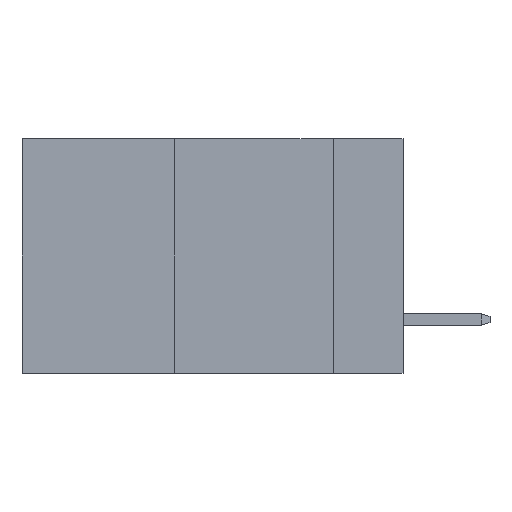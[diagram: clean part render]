
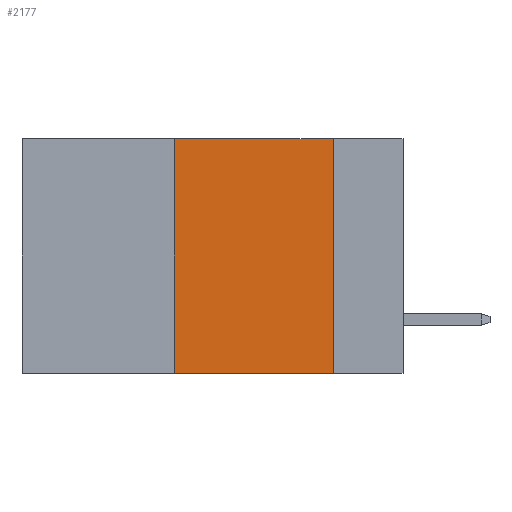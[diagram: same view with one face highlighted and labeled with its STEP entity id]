
A CAD part, left-side view. The second image highlights one B-rep face of the part: STEP entity #2177.
In plain terms, the highlighted planar face has unit normal (-1, 0, 0).
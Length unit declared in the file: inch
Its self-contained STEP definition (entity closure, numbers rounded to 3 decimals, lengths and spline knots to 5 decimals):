
#65 = ORIENTED_EDGE ( 'NONE', *, *, #12275, .F. ) ;
#201 = EDGE_CURVE ( 'NONE', #8243, #3145, #10581, .T. ) ;
#1287 = CARTESIAN_POINT ( 'NONE',  ( 0., 0.36, -0.37 ) ) ;
#1814 = PLANE ( 'NONE',  #11756 ) ;
#1875 = ORIENTED_EDGE ( 'NONE', *, *, #201, .F. ) ;
#1886 = ORIENTED_EDGE ( 'NONE', *, *, #10326, .F. ) ;
#2177 = ADVANCED_FACE ( 'NONE', ( #11460 ), #1814, .F. ) ;
#2230 = EDGE_CURVE ( 'NONE', #8243, #5946, #9363, .T. ) ;
#2442 = CARTESIAN_POINT ( 'NONE',  ( 0., 0.11, 0. ) ) ;
#2740 = VECTOR ( 'NONE', #7527, 39.37008 ) ;
#2976 = CARTESIAN_POINT ( 'NONE',  ( 0., 0.11, 0. ) ) ;
#3145 = VERTEX_POINT ( 'NONE', #3459 ) ;
#3459 = CARTESIAN_POINT ( 'NONE',  ( 0., 0.36, 0. ) ) ;
#4004 = CARTESIAN_POINT ( 'NONE',  ( 0., 0.6, -0.37 ) ) ;
#4870 = ORIENTED_EDGE ( 'NONE', *, *, #2230, .T. ) ;
#4958 = CARTESIAN_POINT ( 'NONE',  ( 0., 0.36, 0. ) ) ;
#5744 = EDGE_LOOP ( 'NONE', ( #65, #1886, #1875, #4870 ) ) ;
#5946 = VERTEX_POINT ( 'NONE', #12658 ) ;
#6119 = CARTESIAN_POINT ( 'NONE',  ( 0., 0.6, 0. ) ) ;
#7527 = DIRECTION ( 'NONE',  ( 0., -1., 0. ) ) ;
#8136 = DIRECTION ( 'NONE',  ( 0., 0., -1. ) ) ;
#8166 = VECTOR ( 'NONE', #8306, 39.37008 ) ;
#8243 = VERTEX_POINT ( 'NONE', #1287 ) ;
#8306 = DIRECTION ( 'NONE',  ( 0., -1., 0. ) ) ;
#8490 = DIRECTION ( 'NONE',  ( 0., 0., 1. ) ) ;
#9363 = LINE ( 'NONE', #4004, #8166 ) ;
#9578 = CARTESIAN_POINT ( 'NONE',  ( 0., 0.6, 0. ) ) ;
#9684 = VECTOR ( 'NONE', #8490, 39.37008 ) ;
#10326 = EDGE_CURVE ( 'NONE', #3145, #12852, #13916, .T. ) ;
#10581 = LINE ( 'NONE', #4958, #9684 ) ;
#11460 = FACE_OUTER_BOUND ( 'NONE', #5744, .T. ) ;
#11756 = AXIS2_PLACEMENT_3D ( 'NONE', #6119, #13719, #13439 ) ;
#12275 = EDGE_CURVE ( 'NONE', #12852, #5946, #12615, .T. ) ;
#12615 = LINE ( 'NONE', #2976, #12644 ) ;
#12644 = VECTOR ( 'NONE', #8136, 39.37008 ) ;
#12658 = CARTESIAN_POINT ( 'NONE',  ( 0., 0.11, -0.37 ) ) ;
#12852 = VERTEX_POINT ( 'NONE', #2442 ) ;
#13439 = DIRECTION ( 'NONE',  ( 0., 0., -1. ) ) ;
#13719 = DIRECTION ( 'NONE',  ( 1., 0., 0. ) ) ;
#13916 = LINE ( 'NONE', #9578, #2740 ) ;
